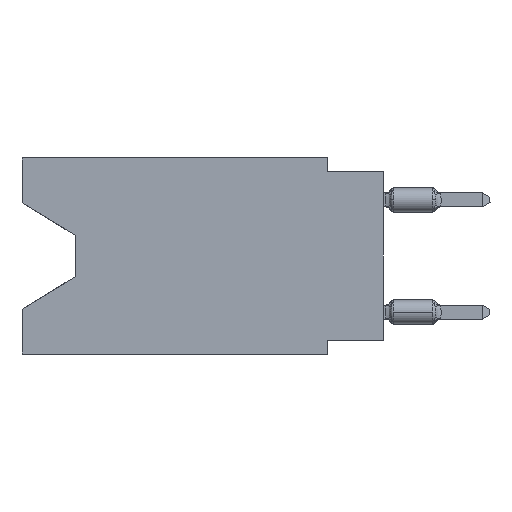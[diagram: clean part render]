
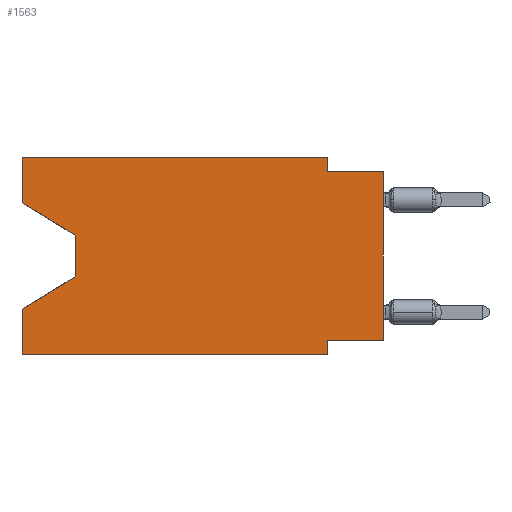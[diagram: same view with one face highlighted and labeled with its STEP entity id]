
A CAD part, left-side view. The second image highlights one B-rep face of the part: STEP entity #1563.
In plain terms, the highlighted planar face has unit normal (-1, 0, 0).
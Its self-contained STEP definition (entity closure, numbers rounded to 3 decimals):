
#304 = CARTESIAN_POINT ( 'NONE',  ( 0., 16.383, -2.038 ) ) ;
#513 = DIRECTION ( 'NONE',  ( 1., 0., 0. ) ) ;
#1563 = ADVANCED_FACE ( 'NONE', ( #16993 ), #2133, .F. ) ;
#1648 = VERTEX_POINT ( 'NONE', #5172 ) ;
#2129 = LINE ( 'NONE', #15754, #6391 ) ;
#2130 = LINE ( 'NONE', #17983, #6913 ) ;
#2133 = PLANE ( 'NONE',  #10543 ) ;
#2238 = VECTOR ( 'NONE', #12945, 1000. ) ;
#2313 = CARTESIAN_POINT ( 'NONE',  ( 0., 2.54, 0. ) ) ;
#2655 = CARTESIAN_POINT ( 'NONE',  ( 0., 2.54, -8.89 ) ) ;
#2679 = DIRECTION ( 'NONE',  ( 0., 1., 0. ) ) ;
#2728 = ORIENTED_EDGE ( 'NONE', *, *, #12373, .F. ) ;
#3264 = CARTESIAN_POINT ( 'NONE',  ( 0., 16.383, -6.852 ) ) ;
#3596 = VECTOR ( 'NONE', #16979, 1000. ) ;
#3899 = DIRECTION ( 'NONE',  ( 0., -1., 0. ) ) ;
#4379 = ORIENTED_EDGE ( 'NONE', *, *, #12925, .T. ) ;
#4431 = VERTEX_POINT ( 'NONE', #18926 ) ;
#5172 = CARTESIAN_POINT ( 'NONE',  ( 0., 0., -8.255 ) ) ;
#5318 = LINE ( 'NONE', #9855, #19655 ) ;
#5423 = ORIENTED_EDGE ( 'NONE', *, *, #9656, .F. ) ;
#5482 = LINE ( 'NONE', #11628, #2238 ) ;
#6391 = VECTOR ( 'NONE', #11313, 1000. ) ;
#6567 = DIRECTION ( 'NONE',  ( 0., -0.855, -0.519 ) ) ;
#6682 = VECTOR ( 'NONE', #7787, 1000. ) ;
#6702 = ORIENTED_EDGE ( 'NONE', *, *, #12504, .F. ) ;
#6845 = LINE ( 'NONE', #12998, #11528 ) ;
#6913 = VECTOR ( 'NONE', #14848, 1000. ) ;
#7174 = CARTESIAN_POINT ( 'NONE',  ( 0., 2.54, -8.255 ) ) ;
#7187 = EDGE_CURVE ( 'NONE', #16246, #14714, #9296, .T. ) ;
#7237 = EDGE_CURVE ( 'NONE', #4431, #8033, #7693, .T. ) ;
#7693 = LINE ( 'NONE', #14133, #3596 ) ;
#7787 = DIRECTION ( 'NONE',  ( 0., -1., 0. ) ) ;
#7815 = EDGE_CURVE ( 'NONE', #1648, #12002, #10352, .T. ) ;
#8032 = CARTESIAN_POINT ( 'NONE',  ( 0., 16.383, 0. ) ) ;
#8033 = VERTEX_POINT ( 'NONE', #3264 ) ;
#8875 = CARTESIAN_POINT ( 'NONE',  ( 0., 13.97, -3.505 ) ) ;
#8936 = VERTEX_POINT ( 'NONE', #11286 ) ;
#9040 = ORIENTED_EDGE ( 'NONE', *, *, #7237, .F. ) ;
#9296 = LINE ( 'NONE', #304, #9728 ) ;
#9656 = EDGE_CURVE ( 'NONE', #16246, #16922, #2130, .T. ) ;
#9728 = VECTOR ( 'NONE', #6567, 1000. ) ;
#9855 = CARTESIAN_POINT ( 'NONE',  ( 0., 16.383, -8.89 ) ) ;
#9893 = CARTESIAN_POINT ( 'NONE',  ( 0., 2.54, -8.89 ) ) ;
#10038 = CARTESIAN_POINT ( 'NONE',  ( 0., 0., 0. ) ) ;
#10352 = LINE ( 'NONE', #16495, #13629 ) ;
#10482 = ORIENTED_EDGE ( 'NONE', *, *, #17452, .F. ) ;
#10543 = AXIS2_PLACEMENT_3D ( 'NONE', #12541, #513, #12632 ) ;
#10812 = ORIENTED_EDGE ( 'NONE', *, *, #7815, .F. ) ;
#11059 = LINE ( 'NONE', #8032, #19268 ) ;
#11286 = CARTESIAN_POINT ( 'NONE',  ( 0., 13.97, -5.385 ) ) ;
#11313 = DIRECTION ( 'NONE',  ( 0., 0.855, -0.519 ) ) ;
#11523 = VERTEX_POINT ( 'NONE', #2655 ) ;
#11528 = VECTOR ( 'NONE', #17645, 1000. ) ;
#11566 = VERTEX_POINT ( 'NONE', #19410 ) ;
#11628 = CARTESIAN_POINT ( 'NONE',  ( 0., 13.97, -3.505 ) ) ;
#11730 = EDGE_CURVE ( 'NONE', #11566, #16081, #15361, .T. ) ;
#12002 = VERTEX_POINT ( 'NONE', #7174 ) ;
#12373 = EDGE_CURVE ( 'NONE', #19794, #11566, #6845, .T. ) ;
#12504 = EDGE_CURVE ( 'NONE', #16922, #19794, #11059, .T. ) ;
#12541 = CARTESIAN_POINT ( 'NONE',  ( 0., 16.383, 0. ) ) ;
#12632 = DIRECTION ( 'NONE',  ( 0., 0., -1. ) ) ;
#12749 = CARTESIAN_POINT ( 'NONE',  ( 0., 16.383, 0. ) ) ;
#12876 = LINE ( 'NONE', #10038, #17735 ) ;
#12925 = EDGE_CURVE ( 'NONE', #8936, #8033, #2129, .T. ) ;
#12945 = DIRECTION ( 'NONE',  ( 0., 0., -1. ) ) ;
#12998 = CARTESIAN_POINT ( 'NONE',  ( 0., 2.54, 0. ) ) ;
#13629 = VECTOR ( 'NONE', #2679, 1000. ) ;
#13894 = DIRECTION ( 'NONE',  ( 0., -1., 0. ) ) ;
#13984 = EDGE_CURVE ( 'NONE', #4431, #11523, #5318, .T. ) ;
#14133 = CARTESIAN_POINT ( 'NONE',  ( 0., 16.383, 0. ) ) ;
#14390 = ORIENTED_EDGE ( 'NONE', *, *, #13984, .T. ) ;
#14714 = VERTEX_POINT ( 'NONE', #8875 ) ;
#14848 = DIRECTION ( 'NONE',  ( 0., 0., 1. ) ) ;
#15088 = ORIENTED_EDGE ( 'NONE', *, *, #7187, .T. ) ;
#15236 = ORIENTED_EDGE ( 'NONE', *, *, #11730, .F. ) ;
#15258 = CARTESIAN_POINT ( 'NONE',  ( 0., 0., -0.635 ) ) ;
#15361 = LINE ( 'NONE', #18195, #6682 ) ;
#15754 = CARTESIAN_POINT ( 'NONE',  ( 0., 13.97, -5.385 ) ) ;
#15847 = EDGE_CURVE ( 'NONE', #14714, #8936, #5482, .T. ) ;
#15896 = VECTOR ( 'NONE', #18979, 1000. ) ;
#16081 = VERTEX_POINT ( 'NONE', #15258 ) ;
#16246 = VERTEX_POINT ( 'NONE', #19591 ) ;
#16495 = CARTESIAN_POINT ( 'NONE',  ( 0., 0., -8.255 ) ) ;
#16679 = EDGE_CURVE ( 'NONE', #1648, #16081, #12876, .T. ) ;
#16922 = VERTEX_POINT ( 'NONE', #12749 ) ;
#16979 = DIRECTION ( 'NONE',  ( 0., 0., 1. ) ) ;
#16993 = FACE_OUTER_BOUND ( 'NONE', #17223, .T. ) ;
#17223 = EDGE_LOOP ( 'NONE', ( #15088, #17426, #4379, #9040, #14390, #10482, #10812, #17612, #15236, #2728, #6702, #5423 ) ) ;
#17375 = LINE ( 'NONE', #9893, #15896 ) ;
#17426 = ORIENTED_EDGE ( 'NONE', *, *, #15847, .T. ) ;
#17452 = EDGE_CURVE ( 'NONE', #12002, #11523, #17375, .T. ) ;
#17612 = ORIENTED_EDGE ( 'NONE', *, *, #16679, .T. ) ;
#17645 = DIRECTION ( 'NONE',  ( 0., 0., -1. ) ) ;
#17735 = VECTOR ( 'NONE', #19026, 1000. ) ;
#17983 = CARTESIAN_POINT ( 'NONE',  ( 0., 16.383, 0. ) ) ;
#18195 = CARTESIAN_POINT ( 'NONE',  ( 0., 0., -0.635 ) ) ;
#18926 = CARTESIAN_POINT ( 'NONE',  ( 0., 16.383, -8.89 ) ) ;
#18979 = DIRECTION ( 'NONE',  ( 0., 0., -1. ) ) ;
#19026 = DIRECTION ( 'NONE',  ( 0., 0., 1. ) ) ;
#19268 = VECTOR ( 'NONE', #13894, 1000. ) ;
#19410 = CARTESIAN_POINT ( 'NONE',  ( 0., 2.54, -0.635 ) ) ;
#19591 = CARTESIAN_POINT ( 'NONE',  ( 0., 16.383, -2.038 ) ) ;
#19655 = VECTOR ( 'NONE', #3899, 1000. ) ;
#19794 = VERTEX_POINT ( 'NONE', #2313 ) ;
